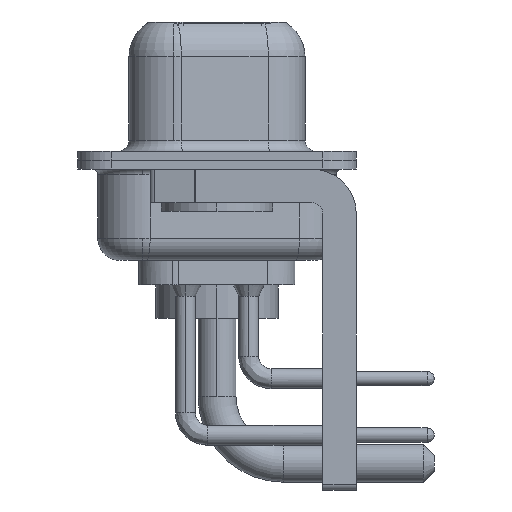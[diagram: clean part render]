
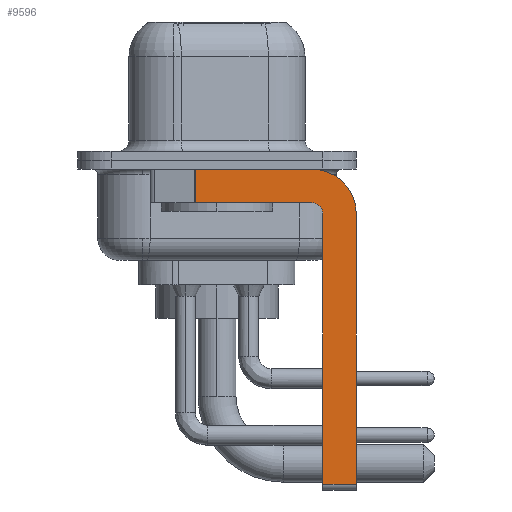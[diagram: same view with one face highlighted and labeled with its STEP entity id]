
A CAD part, left-side view. The second image highlights one B-rep face of the part: STEP entity #9596.
In plain terms, the highlighted planar face has unit normal (-1, 0, 0).
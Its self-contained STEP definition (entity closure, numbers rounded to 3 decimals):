
#190 = VECTOR ( 'NONE', #16831, 1000. ) ;
#213 = CARTESIAN_POINT ( 'NONE',  ( -2.9, 0.978, -0.4 ) ) ;
#225 = CARTESIAN_POINT ( 'NONE',  ( -2.9, -4.25, -1.9 ) ) ;
#563 = ORIENTED_EDGE ( 'NONE', *, *, #831, .F. ) ;
#831 = EDGE_CURVE ( 'NONE', #10580, #18657, #15154, .T. ) ;
#864 = EDGE_CURVE ( 'NONE', #2407, #16413, #18401, .T. ) ;
#1406 = ORIENTED_EDGE ( 'NONE', *, *, #2714, .F. ) ;
#1477 = CARTESIAN_POINT ( 'NONE',  ( -2.9, -6.25, -14.55 ) ) ;
#1659 = DIRECTION ( 'NONE',  ( 0., 0., -1. ) ) ;
#1739 = EDGE_CURVE ( 'NONE', #12984, #12461, #12459, .T. ) ;
#1759 = DIRECTION ( 'NONE',  ( 0., -1., 0. ) ) ;
#2407 = VERTEX_POINT ( 'NONE', #3885 ) ;
#2714 = EDGE_CURVE ( 'NONE', #12461, #10580, #10555, .T. ) ;
#2950 = CARTESIAN_POINT ( 'NONE',  ( -2.9, -4.25, -2.4 ) ) ;
#3039 = ORIENTED_EDGE ( 'NONE', *, *, #864, .F. ) ;
#3053 = EDGE_CURVE ( 'NONE', #6507, #18657, #7117, .T. ) ;
#3162 = CARTESIAN_POINT ( 'NONE',  ( -2.9, -4.75, -2.4 ) ) ;
#3663 = VECTOR ( 'NONE', #12278, 1000. ) ;
#3670 = CARTESIAN_POINT ( 'NONE',  ( -2.9, -4.25, -1.9 ) ) ;
#3885 = CARTESIAN_POINT ( 'NONE',  ( -2.9, -6.25, -2.4 ) ) ;
#4582 = ORIENTED_EDGE ( 'NONE', *, *, #14320, .F. ) ;
#4708 = LINE ( 'NONE', #10705, #16716 ) ;
#4769 = VECTOR ( 'NONE', #19297, 1000. ) ;
#5057 = AXIS2_PLACEMENT_3D ( 'NONE', #2950, #16798, #1659 ) ;
#6175 = VECTOR ( 'NONE', #11724, 1000. ) ;
#6340 = CARTESIAN_POINT ( 'NONE',  ( -2.9, -4.25, -2.4 ) ) ;
#6476 = FACE_OUTER_BOUND ( 'NONE', #6671, .T. ) ;
#6507 = VERTEX_POINT ( 'NONE', #213 ) ;
#6671 = EDGE_LOOP ( 'NONE', ( #15582, #7619, #563, #1406, #15218, #9105, #3039, #4582 ) ) ;
#7019 = AXIS2_PLACEMENT_3D ( 'NONE', #17188, #15311, #12452 ) ;
#7117 = LINE ( 'NONE', #14776, #6175 ) ;
#7161 = VERTEX_POINT ( 'NONE', #14313 ) ;
#7619 = ORIENTED_EDGE ( 'NONE', *, *, #3053, .T. ) ;
#8768 = CARTESIAN_POINT ( 'NONE',  ( -2.9, -4.25, -14.55 ) ) ;
#9001 = DIRECTION ( 'NONE',  ( -1., 0., 0. ) ) ;
#9105 = ORIENTED_EDGE ( 'NONE', *, *, #15039, .T. ) ;
#9445 = DIRECTION ( 'NONE',  ( 0., 1., 0. ) ) ;
#9596 = ADVANCED_FACE ( 'NONE', ( #6476 ), #18655, .F. ) ;
#10555 = CIRCLE ( 'NONE', #13984, 0.5 ) ;
#10580 = VERTEX_POINT ( 'NONE', #3670 ) ;
#10705 = CARTESIAN_POINT ( 'NONE',  ( -2.9, 3., -0.4 ) ) ;
#11337 = CARTESIAN_POINT ( 'NONE',  ( -2.9, -4.75, -14.55 ) ) ;
#11724 = DIRECTION ( 'NONE',  ( 0., 0., -1. ) ) ;
#12137 = DIRECTION ( 'NONE',  ( 0., 0., 1. ) ) ;
#12278 = DIRECTION ( 'NONE',  ( 0., 0., 1. ) ) ;
#12452 = DIRECTION ( 'NONE',  ( 0., 0., -1. ) ) ;
#12459 = LINE ( 'NONE', #15132, #3663 ) ;
#12461 = VERTEX_POINT ( 'NONE', #3162 ) ;
#12476 = CARTESIAN_POINT ( 'NONE',  ( -2.9, -6.25, -2.4 ) ) ;
#12984 = VERTEX_POINT ( 'NONE', #11337 ) ;
#13331 = VECTOR ( 'NONE', #9445, 1000. ) ;
#13984 = AXIS2_PLACEMENT_3D ( 'NONE', #6340, #9001, #12137 ) ;
#14313 = CARTESIAN_POINT ( 'NONE',  ( -2.9, -4.25, -0.4 ) ) ;
#14320 = EDGE_CURVE ( 'NONE', #7161, #2407, #19184, .T. ) ;
#14776 = CARTESIAN_POINT ( 'NONE',  ( -2.9, 0.978, -1.9 ) ) ;
#15039 = EDGE_CURVE ( 'NONE', #12984, #16413, #16233, .T. ) ;
#15132 = CARTESIAN_POINT ( 'NONE',  ( -2.9, -4.75, -14.8 ) ) ;
#15154 = LINE ( 'NONE', #225, #13331 ) ;
#15218 = ORIENTED_EDGE ( 'NONE', *, *, #1739, .F. ) ;
#15311 = DIRECTION ( 'NONE',  ( 1., 0., 0. ) ) ;
#15582 = ORIENTED_EDGE ( 'NONE', *, *, #15635, .F. ) ;
#15635 = EDGE_CURVE ( 'NONE', #6507, #7161, #4708, .T. ) ;
#16233 = LINE ( 'NONE', #8768, #4769 ) ;
#16413 = VERTEX_POINT ( 'NONE', #1477 ) ;
#16716 = VECTOR ( 'NONE', #1759, 1000. ) ;
#16798 = DIRECTION ( 'NONE',  ( 1., 0., 0. ) ) ;
#16831 = DIRECTION ( 'NONE',  ( 0., 0., -1. ) ) ;
#17188 = CARTESIAN_POINT ( 'NONE',  ( -2.9, -4.25, -2.4 ) ) ;
#17415 = CARTESIAN_POINT ( 'NONE',  ( -2.9, 0.978, -1.9 ) ) ;
#18401 = LINE ( 'NONE', #12476, #190 ) ;
#18655 = PLANE ( 'NONE',  #7019 ) ;
#18657 = VERTEX_POINT ( 'NONE', #17415 ) ;
#19184 = CIRCLE ( 'NONE', #5057, 2. ) ;
#19297 = DIRECTION ( 'NONE',  ( 0., -1., 0. ) ) ;
